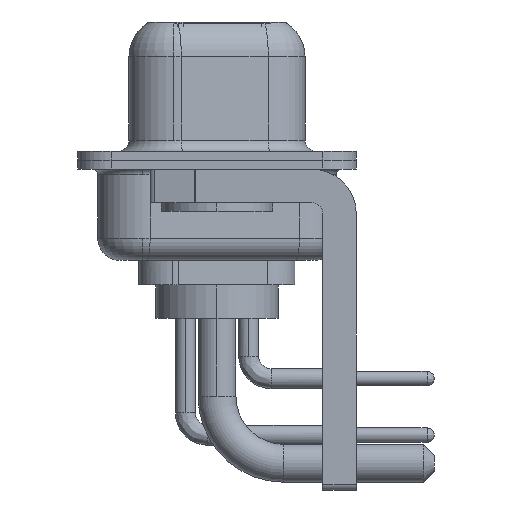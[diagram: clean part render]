
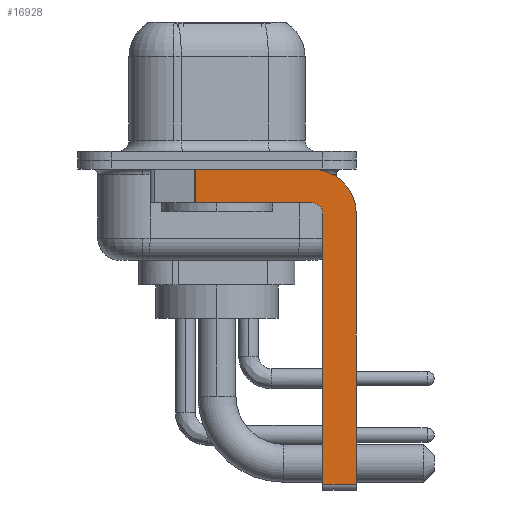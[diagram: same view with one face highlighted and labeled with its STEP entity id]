
A CAD part, left-side view. The second image highlights one B-rep face of the part: STEP entity #16928.
In plain terms, the highlighted planar face has unit normal (-1, 0, 0).
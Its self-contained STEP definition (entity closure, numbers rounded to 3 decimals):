
#93 = VECTOR ( 'NONE', #13316, 1000. ) ;
#333 = FACE_OUTER_BOUND ( 'NONE', #16371, .T. ) ;
#475 = VERTEX_POINT ( 'NONE', #15756 ) ;
#1171 = DIRECTION ( 'NONE',  ( 0., -1., 0. ) ) ;
#1239 = AXIS2_PLACEMENT_3D ( 'NONE', #17419, #17233, #1898 ) ;
#1311 = EDGE_CURVE ( 'NONE', #3012, #2251, #13699, .T. ) ;
#1368 = ORIENTED_EDGE ( 'NONE', *, *, #5246, .F. ) ;
#1898 = DIRECTION ( 'NONE',  ( 0., 0., -1. ) ) ;
#1961 = DIRECTION ( 'NONE',  ( -1., 0., 0. ) ) ;
#2132 = EDGE_CURVE ( 'NONE', #14616, #17148, #10863, .T. ) ;
#2251 = VERTEX_POINT ( 'NONE', #17921 ) ;
#2331 = ORIENTED_EDGE ( 'NONE', *, *, #17245, .F. ) ;
#2432 = ORIENTED_EDGE ( 'NONE', *, *, #8187, .F. ) ;
#2917 = VECTOR ( 'NONE', #6779, 1000. ) ;
#3012 = VERTEX_POINT ( 'NONE', #14530 ) ;
#4987 = DIRECTION ( 'NONE',  ( 0., 0., -1. ) ) ;
#5246 = EDGE_CURVE ( 'NONE', #17148, #16745, #7161, .T. ) ;
#5620 = VECTOR ( 'NONE', #12475, 1000. ) ;
#5678 = LINE ( 'NONE', #12387, #5620 ) ;
#5695 = PLANE ( 'NONE',  #15443 ) ;
#6078 = LINE ( 'NONE', #7732, #7652 ) ;
#6444 = VECTOR ( 'NONE', #1171, 1000. ) ;
#6779 = DIRECTION ( 'NONE',  ( 0., 0., 1. ) ) ;
#7040 = ORIENTED_EDGE ( 'NONE', *, *, #8988, .T. ) ;
#7161 = LINE ( 'NONE', #18027, #14247 ) ;
#7345 = DIRECTION ( 'NONE',  ( 1., 0., 0. ) ) ;
#7652 = VECTOR ( 'NONE', #4987, 1000. ) ;
#7732 = CARTESIAN_POINT ( 'NONE',  ( -2.9, -6.25, -2.4 ) ) ;
#8101 = CARTESIAN_POINT ( 'NONE',  ( -2.9, 3., -0.4 ) ) ;
#8154 = CARTESIAN_POINT ( 'NONE',  ( -2.9, -4.75, -14.8 ) ) ;
#8187 = EDGE_CURVE ( 'NONE', #10362, #17293, #6078, .T. ) ;
#8254 = CARTESIAN_POINT ( 'NONE',  ( -2.9, -6.25, -2.4 ) ) ;
#8266 = EDGE_CURVE ( 'NONE', #2251, #10362, #12046, .T. ) ;
#8560 = ORIENTED_EDGE ( 'NONE', *, *, #8655, .T. ) ;
#8655 = EDGE_CURVE ( 'NONE', #3012, #16745, #17128, .T. ) ;
#8988 = EDGE_CURVE ( 'NONE', #475, #17293, #5678, .T. ) ;
#10182 = CARTESIAN_POINT ( 'NONE',  ( -2.9, -4.25, -2.4 ) ) ;
#10362 = VERTEX_POINT ( 'NONE', #8254 ) ;
#10538 = CARTESIAN_POINT ( 'NONE',  ( -2.9, -4.25, -1.9 ) ) ;
#10863 = CIRCLE ( 'NONE', #12940, 0.5 ) ;
#11742 = DIRECTION ( 'NONE',  ( 0., 0., 1. ) ) ;
#12046 = CIRCLE ( 'NONE', #1239, 2. ) ;
#12116 = ORIENTED_EDGE ( 'NONE', *, *, #1311, .F. ) ;
#12387 = CARTESIAN_POINT ( 'NONE',  ( -2.9, -4.25, -14.55 ) ) ;
#12404 = CARTESIAN_POINT ( 'NONE',  ( -2.9, 0.978, -1.9 ) ) ;
#12475 = DIRECTION ( 'NONE',  ( 0., -1., 0. ) ) ;
#12561 = LINE ( 'NONE', #8154, #2917 ) ;
#12940 = AXIS2_PLACEMENT_3D ( 'NONE', #14483, #1961, #11742 ) ;
#12958 = CARTESIAN_POINT ( 'NONE',  ( -2.9, 0.978, -1.9 ) ) ;
#13316 = DIRECTION ( 'NONE',  ( 0., 0., -1. ) ) ;
#13323 = ORIENTED_EDGE ( 'NONE', *, *, #2132, .F. ) ;
#13699 = LINE ( 'NONE', #8101, #6444 ) ;
#14247 = VECTOR ( 'NONE', #14967, 1000. ) ;
#14483 = CARTESIAN_POINT ( 'NONE',  ( -2.9, -4.25, -2.4 ) ) ;
#14530 = CARTESIAN_POINT ( 'NONE',  ( -2.9, 0.978, -0.4 ) ) ;
#14616 = VERTEX_POINT ( 'NONE', #17625 ) ;
#14967 = DIRECTION ( 'NONE',  ( 0., 1., 0. ) ) ;
#15443 = AXIS2_PLACEMENT_3D ( 'NONE', #10182, #7345, #17037 ) ;
#15756 = CARTESIAN_POINT ( 'NONE',  ( -2.9, -4.75, -14.55 ) ) ;
#16022 = ORIENTED_EDGE ( 'NONE', *, *, #8266, .F. ) ;
#16371 = EDGE_LOOP ( 'NONE', ( #12116, #8560, #1368, #13323, #2331, #7040, #2432, #16022 ) ) ;
#16745 = VERTEX_POINT ( 'NONE', #12404 ) ;
#16928 = ADVANCED_FACE ( 'NONE', ( #333 ), #5695, .F. ) ;
#17037 = DIRECTION ( 'NONE',  ( 0., 0., -1. ) ) ;
#17128 = LINE ( 'NONE', #12958, #93 ) ;
#17148 = VERTEX_POINT ( 'NONE', #10538 ) ;
#17233 = DIRECTION ( 'NONE',  ( 1., 0., 0. ) ) ;
#17245 = EDGE_CURVE ( 'NONE', #475, #14616, #12561, .T. ) ;
#17293 = VERTEX_POINT ( 'NONE', #17751 ) ;
#17419 = CARTESIAN_POINT ( 'NONE',  ( -2.9, -4.25, -2.4 ) ) ;
#17625 = CARTESIAN_POINT ( 'NONE',  ( -2.9, -4.75, -2.4 ) ) ;
#17751 = CARTESIAN_POINT ( 'NONE',  ( -2.9, -6.25, -14.55 ) ) ;
#17921 = CARTESIAN_POINT ( 'NONE',  ( -2.9, -4.25, -0.4 ) ) ;
#18027 = CARTESIAN_POINT ( 'NONE',  ( -2.9, -4.25, -1.9 ) ) ;
